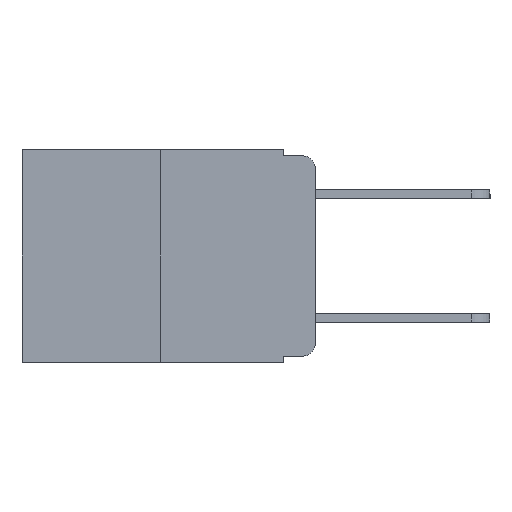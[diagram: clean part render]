
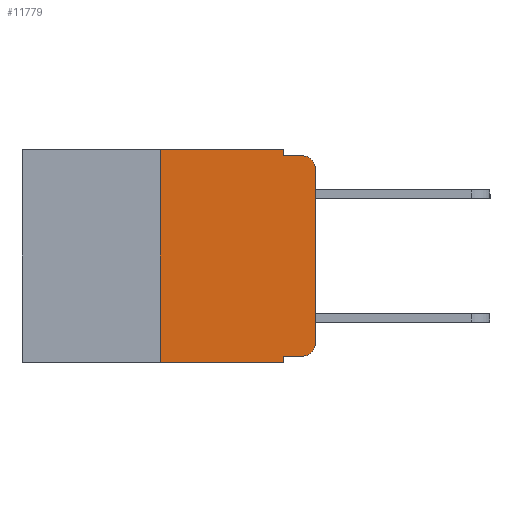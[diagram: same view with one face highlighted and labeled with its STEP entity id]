
A CAD part, left-side view. The second image highlights one B-rep face of the part: STEP entity #11779.
In plain terms, the highlighted planar face has unit normal (-1, 0, 0).
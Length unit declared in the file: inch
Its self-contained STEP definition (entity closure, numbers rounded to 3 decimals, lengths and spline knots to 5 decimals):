
#37 = VECTOR ( 'NONE', #1618, 39.37008 ) ;
#218 = DIRECTION ( 'NONE',  ( 0., -1., 0. ) ) ;
#559 = CARTESIAN_POINT ( 'NONE',  ( 0., 0.473, 0. ) ) ;
#887 = VERTEX_POINT ( 'NONE', #8985 ) ;
#1064 = VERTEX_POINT ( 'NONE', #1210 ) ;
#1195 = VERTEX_POINT ( 'NONE', #3361 ) ;
#1210 = CARTESIAN_POINT ( 'NONE',  ( 0., 0., -0.313 ) ) ;
#1224 = DIRECTION ( 'NONE',  ( 1., 0., 0. ) ) ;
#1550 = CARTESIAN_POINT ( 'NONE',  ( 0., 0.051, 0. ) ) ;
#1618 = DIRECTION ( 'NONE',  ( 0., 0., 1. ) ) ;
#1987 = LINE ( 'NONE', #10682, #4986 ) ;
#2173 = VERTEX_POINT ( 'NONE', #1550 ) ;
#3323 = DIRECTION ( 'NONE',  ( -1., 0., 0. ) ) ;
#3361 = CARTESIAN_POINT ( 'NONE',  ( 0., 0., -0.03 ) ) ;
#3631 = CARTESIAN_POINT ( 'NONE',  ( 0., 0.25, 0. ) ) ;
#3803 = EDGE_LOOP ( 'NONE', ( #5254, #5004, #11360, #12242, #11980, #11611, #11164, #5326, #5139, #12687 ) ) ;
#3894 = CARTESIAN_POINT ( 'NONE',  ( 0., 0.051, -0.01 ) ) ;
#3967 = VERTEX_POINT ( 'NONE', #12009 ) ;
#4200 = AXIS2_PLACEMENT_3D ( 'NONE', #9086, #3323, #10011 ) ;
#4246 = VERTEX_POINT ( 'NONE', #11471 ) ;
#4593 = LINE ( 'NONE', #3894, #6858 ) ;
#4723 = LINE ( 'NONE', #12181, #9679 ) ;
#4986 = VECTOR ( 'NONE', #6157, 39.37008 ) ;
#4996 = CARTESIAN_POINT ( 'NONE',  ( 0., 0., 0. ) ) ;
#5004 = ORIENTED_EDGE ( 'NONE', *, *, #8433, .T. ) ;
#5060 = DIRECTION ( 'NONE',  ( 0., -1., 0. ) ) ;
#5139 = ORIENTED_EDGE ( 'NONE', *, *, #5428, .T. ) ;
#5164 = EDGE_CURVE ( 'NONE', #6173, #4246, #4723, .T. ) ;
#5254 = ORIENTED_EDGE ( 'NONE', *, *, #10709, .T. ) ;
#5307 = AXIS2_PLACEMENT_3D ( 'NONE', #11877, #6546, #12715 ) ;
#5326 = ORIENTED_EDGE ( 'NONE', *, *, #5164, .F. ) ;
#5428 = EDGE_CURVE ( 'NONE', #6173, #5780, #8271, .T. ) ;
#5434 = AXIS2_PLACEMENT_3D ( 'NONE', #9336, #1224, #8470 ) ;
#5461 = DIRECTION ( 'NONE',  ( 0., -1., 0. ) ) ;
#5780 = VERTEX_POINT ( 'NONE', #7391 ) ;
#5815 = EDGE_CURVE ( 'NONE', #5780, #1064, #7973, .T. ) ;
#6103 = LINE ( 'NONE', #4996, #37 ) ;
#6157 = DIRECTION ( 'NONE',  ( 0., 0., -1. ) ) ;
#6173 = VERTEX_POINT ( 'NONE', #9854 ) ;
#6176 = CIRCLE ( 'NONE', #4200, 0.02 ) ;
#6546 = DIRECTION ( 'NONE',  ( -1., 0., 0. ) ) ;
#6858 = VECTOR ( 'NONE', #218, 39.37008 ) ;
#7391 = CARTESIAN_POINT ( 'NONE',  ( 0., 0.02, -0.333 ) ) ;
#7661 = EDGE_CURVE ( 'NONE', #2173, #887, #1987, .T. ) ;
#7919 = LINE ( 'NONE', #559, #12030 ) ;
#7973 = CIRCLE ( 'NONE', #5307, 0.02 ) ;
#8223 = CARTESIAN_POINT ( 'NONE',  ( 0., 0.473, -0.343 ) ) ;
#8271 = LINE ( 'NONE', #11426, #11578 ) ;
#8310 = EDGE_CURVE ( 'NONE', #11489, #2173, #7919, .T. ) ;
#8433 = EDGE_CURVE ( 'NONE', #1195, #3967, #6176, .T. ) ;
#8470 = DIRECTION ( 'NONE',  ( 0., 0., -1. ) ) ;
#8697 = VECTOR ( 'NONE', #10238, 39.37008 ) ;
#8777 = LINE ( 'NONE', #8223, #10879 ) ;
#8850 = DIRECTION ( 'NONE',  ( 0., -1., 0. ) ) ;
#8985 = CARTESIAN_POINT ( 'NONE',  ( 0., 0.051, -0.01 ) ) ;
#9086 = CARTESIAN_POINT ( 'NONE',  ( 0., 0.02, -0.03 ) ) ;
#9336 = CARTESIAN_POINT ( 'NONE',  ( 0., 0.473, 0. ) ) ;
#9480 = EDGE_CURVE ( 'NONE', #887, #3967, #4593, .T. ) ;
#9679 = VECTOR ( 'NONE', #11401, 39.37008 ) ;
#9854 = CARTESIAN_POINT ( 'NONE',  ( 0., 0.051, -0.333 ) ) ;
#9931 = FACE_OUTER_BOUND ( 'NONE', #3803, .T. ) ;
#10011 = DIRECTION ( 'NONE',  ( 0., 0., -1. ) ) ;
#10238 = DIRECTION ( 'NONE',  ( 0., 0., 1. ) ) ;
#10530 = EDGE_CURVE ( 'NONE', #11455, #11489, #10799, .T. ) ;
#10682 = CARTESIAN_POINT ( 'NONE',  ( 0., 0.051, 0. ) ) ;
#10709 = EDGE_CURVE ( 'NONE', #1064, #1195, #6103, .T. ) ;
#10799 = LINE ( 'NONE', #3631, #8697 ) ;
#10879 = VECTOR ( 'NONE', #5461, 39.37008 ) ;
#11115 = PLANE ( 'NONE',  #5434 ) ;
#11164 = ORIENTED_EDGE ( 'NONE', *, *, #12731, .T. ) ;
#11360 = ORIENTED_EDGE ( 'NONE', *, *, #9480, .F. ) ;
#11401 = DIRECTION ( 'NONE',  ( 0., 0., -1. ) ) ;
#11426 = CARTESIAN_POINT ( 'NONE',  ( 0., 0.051, -0.333 ) ) ;
#11455 = VERTEX_POINT ( 'NONE', #12293 ) ;
#11471 = CARTESIAN_POINT ( 'NONE',  ( 0., 0.051, -0.343 ) ) ;
#11489 = VERTEX_POINT ( 'NONE', #11505 ) ;
#11505 = CARTESIAN_POINT ( 'NONE',  ( 0., 0.25, 0. ) ) ;
#11578 = VECTOR ( 'NONE', #5060, 39.37008 ) ;
#11611 = ORIENTED_EDGE ( 'NONE', *, *, #10530, .F. ) ;
#11779 = ADVANCED_FACE ( 'NONE', ( #9931 ), #11115, .F. ) ;
#11877 = CARTESIAN_POINT ( 'NONE',  ( 0., 0.02, -0.313 ) ) ;
#11980 = ORIENTED_EDGE ( 'NONE', *, *, #8310, .F. ) ;
#12009 = CARTESIAN_POINT ( 'NONE',  ( 0., 0.02, -0.01 ) ) ;
#12030 = VECTOR ( 'NONE', #8850, 39.37008 ) ;
#12181 = CARTESIAN_POINT ( 'NONE',  ( 0., 0.051, 0. ) ) ;
#12242 = ORIENTED_EDGE ( 'NONE', *, *, #7661, .F. ) ;
#12293 = CARTESIAN_POINT ( 'NONE',  ( 0., 0.25, -0.343 ) ) ;
#12687 = ORIENTED_EDGE ( 'NONE', *, *, #5815, .T. ) ;
#12715 = DIRECTION ( 'NONE',  ( 0., 0., -1. ) ) ;
#12731 = EDGE_CURVE ( 'NONE', #11455, #4246, #8777, .T. ) ;
